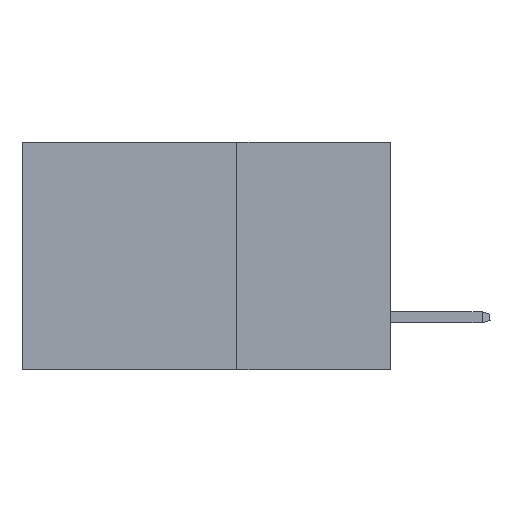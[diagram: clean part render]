
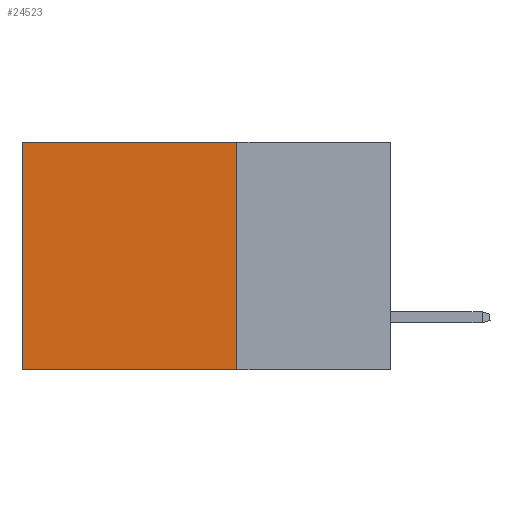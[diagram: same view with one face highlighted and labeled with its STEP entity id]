
A CAD part, left-side view. The second image highlights one B-rep face of the part: STEP entity #24523.
In plain terms, the highlighted planar face has unit normal (-1, 0, 0).
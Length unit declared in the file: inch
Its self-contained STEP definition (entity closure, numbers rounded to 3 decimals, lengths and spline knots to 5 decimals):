
#131 = LINE ( 'NONE', #18537, #15304 ) ;
#222 = DIRECTION ( 'NONE',  ( 0., 0., -1. ) ) ;
#264 = VERTEX_POINT ( 'NONE', #6945 ) ;
#975 = VECTOR ( 'NONE', #9968, 39.37008 ) ;
#2736 = DIRECTION ( 'NONE',  ( 1., 0., 0. ) ) ;
#3037 = EDGE_CURVE ( 'NONE', #13973, #17772, #131, .T. ) ;
#3345 = VECTOR ( 'NONE', #22926, 39.37008 ) ;
#6181 = VECTOR ( 'NONE', #9456, 39.37008 ) ;
#6945 = CARTESIAN_POINT ( 'NONE',  ( 0.2875, 0.25, 0. ) ) ;
#7050 = CARTESIAN_POINT ( 'NONE',  ( 0.2875, 0.25, 0. ) ) ;
#7930 = CARTESIAN_POINT ( 'NONE',  ( 0.2875, 0.25, -0.37 ) ) ;
#9179 = CARTESIAN_POINT ( 'NONE',  ( 0.2875, 0.6, -0.37 ) ) ;
#9369 = EDGE_CURVE ( 'NONE', #264, #10247, #13817, .T. ) ;
#9456 = DIRECTION ( 'NONE',  ( 0., 1., 0. ) ) ;
#9642 = EDGE_CURVE ( 'NONE', #264, #13973, #21238, .T. ) ;
#9968 = DIRECTION ( 'NONE',  ( 0., 1., 0. ) ) ;
#10247 = VERTEX_POINT ( 'NONE', #21671 ) ;
#12046 = ORIENTED_EDGE ( 'NONE', *, *, #9369, .F. ) ;
#12706 = FACE_OUTER_BOUND ( 'NONE', #24608, .T. ) ;
#12937 = PLANE ( 'NONE',  #20916 ) ;
#13817 = LINE ( 'NONE', #25240, #3345 ) ;
#13973 = VERTEX_POINT ( 'NONE', #21788 ) ;
#15059 = EDGE_CURVE ( 'NONE', #10247, #17772, #17754, .T. ) ;
#15304 = VECTOR ( 'NONE', #222, 39.37008 ) ;
#15829 = ORIENTED_EDGE ( 'NONE', *, *, #3037, .T. ) ;
#17127 = CARTESIAN_POINT ( 'NONE',  ( 0.2875, 0.25, 0. ) ) ;
#17745 = ORIENTED_EDGE ( 'NONE', *, *, #15059, .F. ) ;
#17754 = LINE ( 'NONE', #7930, #975 ) ;
#17772 = VERTEX_POINT ( 'NONE', #9179 ) ;
#18537 = CARTESIAN_POINT ( 'NONE',  ( 0.2875, 0.6, 0. ) ) ;
#18852 = DIRECTION ( 'NONE',  ( 0., 0., -1. ) ) ;
#20916 = AXIS2_PLACEMENT_3D ( 'NONE', #7050, #2736, #18852 ) ;
#21034 = ORIENTED_EDGE ( 'NONE', *, *, #9642, .T. ) ;
#21238 = LINE ( 'NONE', #17127, #6181 ) ;
#21671 = CARTESIAN_POINT ( 'NONE',  ( 0.2875, 0.25, -0.37 ) ) ;
#21788 = CARTESIAN_POINT ( 'NONE',  ( 0.2875, 0.6, 0. ) ) ;
#22926 = DIRECTION ( 'NONE',  ( 0., 0., -1. ) ) ;
#24523 = ADVANCED_FACE ( 'NONE', ( #12706 ), #12937, .F. ) ;
#24608 = EDGE_LOOP ( 'NONE', ( #15829, #17745, #12046, #21034 ) ) ;
#25240 = CARTESIAN_POINT ( 'NONE',  ( 0.2875, 0.25, 0. ) ) ;
